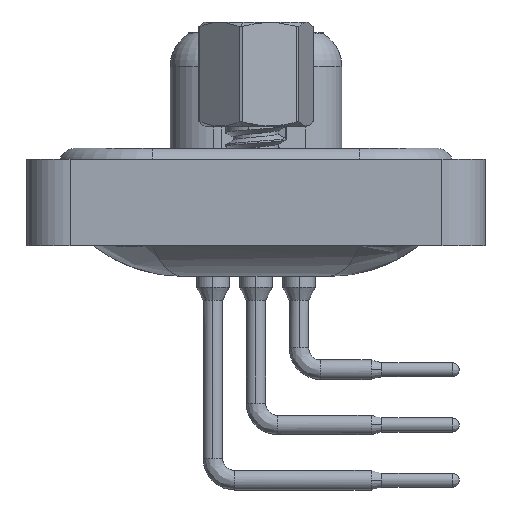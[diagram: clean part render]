
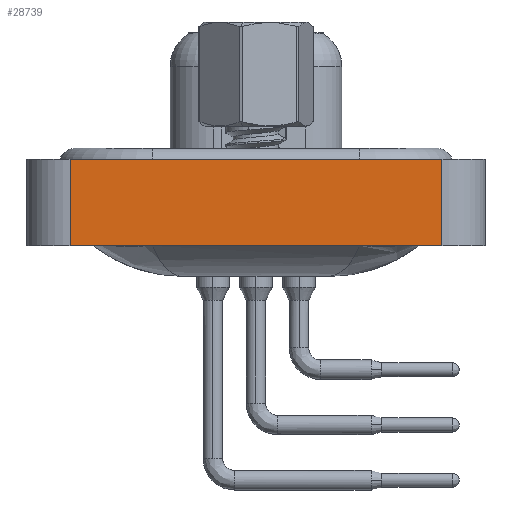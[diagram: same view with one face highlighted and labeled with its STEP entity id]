
A CAD part, left-side view. The second image highlights one B-rep face of the part: STEP entity #28739.
In plain terms, the highlighted planar face has unit normal (-1, 0, 0).
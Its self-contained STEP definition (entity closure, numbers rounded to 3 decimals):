
#238 = CARTESIAN_POINT ( 'NONE',  ( -7.285, -8.55, 0.4 ) ) ;
#1009 = ORIENTED_EDGE ( 'NONE', *, *, #2103, .F. ) ;
#1946 = LINE ( 'NONE', #30496, #29560 ) ;
#2103 = EDGE_CURVE ( 'NONE', #29959, #23783, #12094, .T. ) ;
#2340 = VECTOR ( 'NONE', #29492, 1000. ) ;
#2551 = DIRECTION ( 'NONE',  ( 0., 0., 1. ) ) ;
#3005 = VERTEX_POINT ( 'NONE', #3103 ) ;
#3103 = CARTESIAN_POINT ( 'NONE',  ( -7.285, 8.55, -3.6 ) ) ;
#3643 = ORIENTED_EDGE ( 'NONE', *, *, #24505, .F. ) ;
#3777 = AXIS2_PLACEMENT_3D ( 'NONE', #4595, #9560, #2551 ) ;
#4270 = ORIENTED_EDGE ( 'NONE', *, *, #7846, .T. ) ;
#4595 = CARTESIAN_POINT ( 'NONE',  ( -7.285, -8.55, -3.6 ) ) ;
#6947 = DIRECTION ( 'NONE',  ( 0., 0., 1. ) ) ;
#7222 = FACE_OUTER_BOUND ( 'NONE', #15310, .T. ) ;
#7846 = EDGE_CURVE ( 'NONE', #8014, #23783, #1946, .T. ) ;
#8014 = VERTEX_POINT ( 'NONE', #27031 ) ;
#9560 = DIRECTION ( 'NONE',  ( -1., 0., 0. ) ) ;
#9879 = LINE ( 'NONE', #29517, #20230 ) ;
#11882 = VECTOR ( 'NONE', #23615, 1000. ) ;
#12094 = LINE ( 'NONE', #238, #11882 ) ;
#13353 = CARTESIAN_POINT ( 'NONE',  ( -7.285, 8.55, 0.4 ) ) ;
#14688 = PLANE ( 'NONE',  #3777 ) ;
#15310 = EDGE_LOOP ( 'NONE', ( #4270, #1009, #3643, #27032 ) ) ;
#15974 = EDGE_CURVE ( 'NONE', #3005, #8014, #9879, .T. ) ;
#17018 = LINE ( 'NONE', #24344, #2340 ) ;
#20230 = VECTOR ( 'NONE', #21697, 1000. ) ;
#21697 = DIRECTION ( 'NONE',  ( 0., -1., 0. ) ) ;
#23615 = DIRECTION ( 'NONE',  ( 0., -1., 0. ) ) ;
#23783 = VERTEX_POINT ( 'NONE', #26802 ) ;
#24344 = CARTESIAN_POINT ( 'NONE',  ( -7.285, 8.55, -3.6 ) ) ;
#24505 = EDGE_CURVE ( 'NONE', #3005, #29959, #17018, .T. ) ;
#26802 = CARTESIAN_POINT ( 'NONE',  ( -7.285, -8.55, 0.4 ) ) ;
#27031 = CARTESIAN_POINT ( 'NONE',  ( -7.285, -8.55, -3.6 ) ) ;
#27032 = ORIENTED_EDGE ( 'NONE', *, *, #15974, .T. ) ;
#28739 = ADVANCED_FACE ( 'NONE', ( #7222 ), #14688, .T. ) ;
#29492 = DIRECTION ( 'NONE',  ( 0., 0., 1. ) ) ;
#29517 = CARTESIAN_POINT ( 'NONE',  ( -7.285, -8.55, -3.6 ) ) ;
#29560 = VECTOR ( 'NONE', #6947, 1000. ) ;
#29959 = VERTEX_POINT ( 'NONE', #13353 ) ;
#30496 = CARTESIAN_POINT ( 'NONE',  ( -7.285, -8.55, -3.6 ) ) ;
